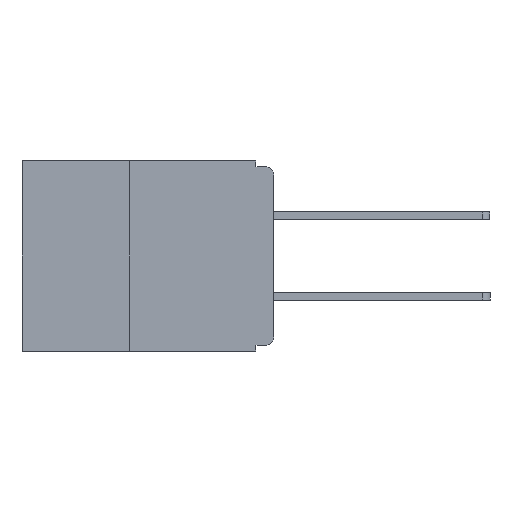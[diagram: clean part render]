
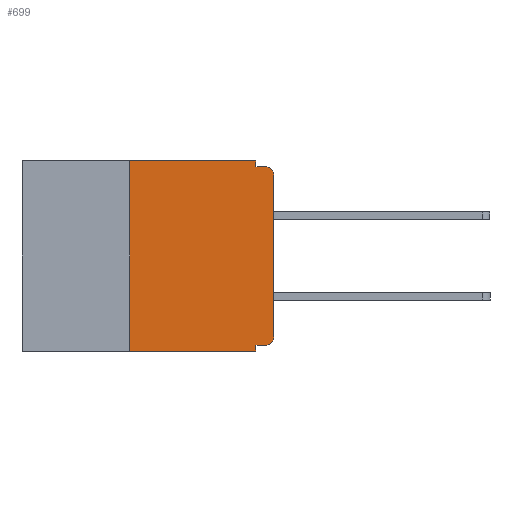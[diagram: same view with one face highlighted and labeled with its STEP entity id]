
A CAD part, left-side view. The second image highlights one B-rep face of the part: STEP entity #699.
In plain terms, the highlighted planar face has unit normal (-1, 0, 0).
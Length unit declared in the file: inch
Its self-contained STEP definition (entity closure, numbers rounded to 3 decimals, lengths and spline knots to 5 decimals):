
#221 = LINE ( 'NONE', #12747, #23869 ) ;
#699 = ADVANCED_FACE ( 'NONE', ( #6827 ), #9343, .F. ) ;
#1318 = CARTESIAN_POINT ( 'NONE',  ( 0., 0.031, -0.32 ) ) ;
#1696 = CARTESIAN_POINT ( 'NONE',  ( 0., 0.031, -0.01 ) ) ;
#1791 = CARTESIAN_POINT ( 'NONE',  ( 0., 0.031, 0. ) ) ;
#2555 = CARTESIAN_POINT ( 'NONE',  ( 0., 0., 0. ) ) ;
#3467 = ORIENTED_EDGE ( 'NONE', *, *, #17710, .F. ) ;
#3919 = CARTESIAN_POINT ( 'NONE',  ( 0., 0.015, -0.01 ) ) ;
#4128 = LINE ( 'NONE', #22359, #15599 ) ;
#4222 = VECTOR ( 'NONE', #5557, 39.37008 ) ;
#4922 = DIRECTION ( 'NONE',  ( 0., 0., 1. ) ) ;
#5072 = VERTEX_POINT ( 'NONE', #1791 ) ;
#5114 = VERTEX_POINT ( 'NONE', #1318 ) ;
#5172 = DIRECTION ( 'NONE',  ( -1., 0., 0. ) ) ;
#5539 = CARTESIAN_POINT ( 'NONE',  ( 0., 0., -0.025 ) ) ;
#5557 = DIRECTION ( 'NONE',  ( 0., -1., 0. ) ) ;
#5800 = DIRECTION ( 'NONE',  ( -1., 0., 0. ) ) ;
#6724 = VECTOR ( 'NONE', #9626, 39.37008 ) ;
#6827 = FACE_OUTER_BOUND ( 'NONE', #27092, .T. ) ;
#7433 = LINE ( 'NONE', #16379, #6724 ) ;
#7882 = LINE ( 'NONE', #21974, #25287 ) ;
#7978 = VERTEX_POINT ( 'NONE', #26609 ) ;
#8856 = EDGE_CURVE ( 'NONE', #23630, #20883, #26643, .T. ) ;
#9156 = VERTEX_POINT ( 'NONE', #3919 ) ;
#9343 = PLANE ( 'NONE',  #23749 ) ;
#9570 = LINE ( 'NONE', #2555, #26865 ) ;
#9626 = DIRECTION ( 'NONE',  ( 0., -1., 0. ) ) ;
#9721 = DIRECTION ( 'NONE',  ( 0., 1., 0. ) ) ;
#9788 = ORIENTED_EDGE ( 'NONE', *, *, #23391, .T. ) ;
#9869 = DIRECTION ( 'NONE',  ( 0., 0., -1. ) ) ;
#9889 = CARTESIAN_POINT ( 'NONE',  ( 0., 0.25, 0. ) ) ;
#10001 = DIRECTION ( 'NONE',  ( 1., 0., 0. ) ) ;
#10111 = ORIENTED_EDGE ( 'NONE', *, *, #14805, .F. ) ;
#10608 = CIRCLE ( 'NONE', #27926, 0.015 ) ;
#11270 = VERTEX_POINT ( 'NONE', #1696 ) ;
#11721 = CARTESIAN_POINT ( 'NONE',  ( 0., 0.437, 0. ) ) ;
#12085 = LINE ( 'NONE', #18859, #16709 ) ;
#12498 = CARTESIAN_POINT ( 'NONE',  ( 0., 0.015, -0.32 ) ) ;
#12614 = LINE ( 'NONE', #29327, #23263 ) ;
#12729 = ORIENTED_EDGE ( 'NONE', *, *, #20942, .F. ) ;
#12747 = CARTESIAN_POINT ( 'NONE',  ( 0., 0.25, -0.33 ) ) ;
#12819 = DIRECTION ( 'NONE',  ( 0., 0., -1. ) ) ;
#13858 = EDGE_CURVE ( 'NONE', #11270, #9156, #12614, .T. ) ;
#13871 = VERTEX_POINT ( 'NONE', #23037 ) ;
#13991 = ORIENTED_EDGE ( 'NONE', *, *, #29207, .T. ) ;
#14047 = ORIENTED_EDGE ( 'NONE', *, *, #22047, .T. ) ;
#14805 = EDGE_CURVE ( 'NONE', #7978, #16784, #221, .T. ) ;
#15599 = VECTOR ( 'NONE', #28953, 39.37008 ) ;
#15821 = EDGE_CURVE ( 'NONE', #16784, #5072, #7433, .T. ) ;
#15907 = EDGE_CURVE ( 'NONE', #23630, #5114, #12085, .T. ) ;
#16379 = CARTESIAN_POINT ( 'NONE',  ( 0., 0.437, 0. ) ) ;
#16709 = VECTOR ( 'NONE', #9721, 39.37008 ) ;
#16784 = VERTEX_POINT ( 'NONE', #9889 ) ;
#17710 = EDGE_CURVE ( 'NONE', #5072, #11270, #4128, .T. ) ;
#18837 = CARTESIAN_POINT ( 'NONE',  ( 0., 0.015, -0.305 ) ) ;
#18859 = CARTESIAN_POINT ( 'NONE',  ( 0., 0., -0.32 ) ) ;
#19501 = CARTESIAN_POINT ( 'NONE',  ( 0., 0.015, -0.025 ) ) ;
#19518 = CARTESIAN_POINT ( 'NONE',  ( 0., 0., -0.305 ) ) ;
#20667 = DIRECTION ( 'NONE',  ( 0., -1., 0. ) ) ;
#20883 = VERTEX_POINT ( 'NONE', #19518 ) ;
#20942 = EDGE_CURVE ( 'NONE', #5114, #13871, #7882, .T. ) ;
#21114 = DIRECTION ( 'NONE',  ( 0., 0., -1. ) ) ;
#21509 = CARTESIAN_POINT ( 'NONE',  ( 0., 0.437, -0.33 ) ) ;
#21760 = DIRECTION ( 'NONE',  ( 0., 0., -1. ) ) ;
#21974 = CARTESIAN_POINT ( 'NONE',  ( 0., 0.031, -0.33 ) ) ;
#22047 = EDGE_CURVE ( 'NONE', #7978, #13871, #28306, .T. ) ;
#22359 = CARTESIAN_POINT ( 'NONE',  ( 0., 0.031, 0. ) ) ;
#23037 = CARTESIAN_POINT ( 'NONE',  ( 0., 0.031, -0.33 ) ) ;
#23263 = VECTOR ( 'NONE', #20667, 39.37008 ) ;
#23391 = EDGE_CURVE ( 'NONE', #20883, #24776, #9570, .T. ) ;
#23630 = VERTEX_POINT ( 'NONE', #12498 ) ;
#23749 = AXIS2_PLACEMENT_3D ( 'NONE', #11721, #10001, #9869 ) ;
#23869 = VECTOR ( 'NONE', #26266, 39.37008 ) ;
#24776 = VERTEX_POINT ( 'NONE', #5539 ) ;
#25054 = ORIENTED_EDGE ( 'NONE', *, *, #8856, .T. ) ;
#25287 = VECTOR ( 'NONE', #12819, 39.37008 ) ;
#26266 = DIRECTION ( 'NONE',  ( 0., 0., 1. ) ) ;
#26609 = CARTESIAN_POINT ( 'NONE',  ( 0., 0.25, -0.33 ) ) ;
#26643 = CIRCLE ( 'NONE', #26665, 0.015 ) ;
#26645 = ORIENTED_EDGE ( 'NONE', *, *, #13858, .F. ) ;
#26665 = AXIS2_PLACEMENT_3D ( 'NONE', #18837, #5172, #21114 ) ;
#26769 = ORIENTED_EDGE ( 'NONE', *, *, #15907, .F. ) ;
#26836 = ORIENTED_EDGE ( 'NONE', *, *, #15821, .F. ) ;
#26865 = VECTOR ( 'NONE', #4922, 39.37008 ) ;
#27092 = EDGE_LOOP ( 'NONE', ( #9788, #13991, #26645, #3467, #26836, #10111, #14047, #12729, #26769, #25054 ) ) ;
#27926 = AXIS2_PLACEMENT_3D ( 'NONE', #19501, #5800, #21760 ) ;
#28306 = LINE ( 'NONE', #21509, #4222 ) ;
#28953 = DIRECTION ( 'NONE',  ( 0., 0., -1. ) ) ;
#29207 = EDGE_CURVE ( 'NONE', #24776, #9156, #10608, .T. ) ;
#29327 = CARTESIAN_POINT ( 'NONE',  ( 0., 0., -0.01 ) ) ;
